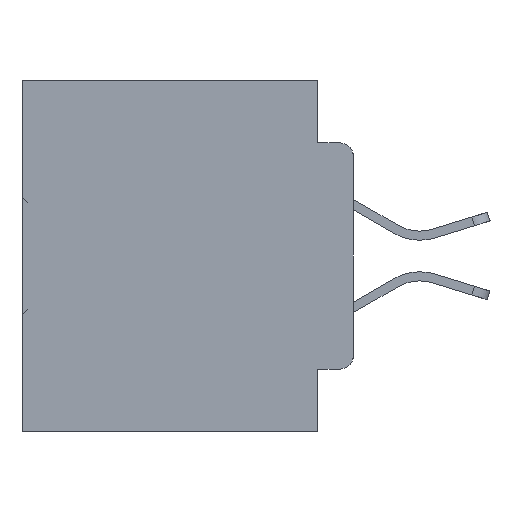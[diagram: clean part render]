
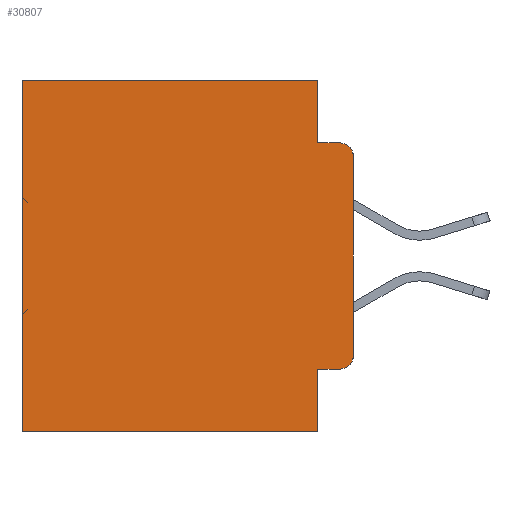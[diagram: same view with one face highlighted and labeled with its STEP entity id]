
A CAD part, left-side view. The second image highlights one B-rep face of the part: STEP entity #30807.
In plain terms, the highlighted planar face has unit normal (-1, 0, 0).
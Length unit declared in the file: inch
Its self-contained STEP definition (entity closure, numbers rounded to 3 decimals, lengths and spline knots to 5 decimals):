
#446 = CARTESIAN_POINT ( 'NONE',  ( 0.298, 0.051, -0.4115 ) ) ;
#1013 = VERTEX_POINT ( 'NONE', #8105 ) ;
#1316 = DIRECTION ( 'NONE',  ( 1., 0., 0. ) ) ;
#1449 = VECTOR ( 'NONE', #35092, 39.37008 ) ;
#1541 = EDGE_CURVE ( 'NONE', #20208, #4711, #32764, .T. ) ;
#1585 = VERTEX_POINT ( 'NONE', #5259 ) ;
#3361 = ORIENTED_EDGE ( 'NONE', *, *, #20859, .T. ) ;
#3576 = VECTOR ( 'NONE', #9005, 39.37008 ) ;
#4711 = VERTEX_POINT ( 'NONE', #33157 ) ;
#5133 = DIRECTION ( 'NONE',  ( 0., 1., 0. ) ) ;
#5152 = AXIS2_PLACEMENT_3D ( 'NONE', #24605, #1316, #24485 ) ;
#5259 = CARTESIAN_POINT ( 'NONE',  ( 0.298, 0.473, -0.5 ) ) ;
#5609 = VERTEX_POINT ( 'NONE', #18625 ) ;
#5916 = VECTOR ( 'NONE', #22371, 39.37008 ) ;
#7751 = LINE ( 'NONE', #8221, #5916 ) ;
#8022 = LINE ( 'NONE', #22755, #19784 ) ;
#8098 = EDGE_LOOP ( 'NONE', ( #30138, #3361, #35336, #16596, #19756, #23698, #16095, #12372, #8615, #29081 ) ) ;
#8105 = CARTESIAN_POINT ( 'NONE',  ( 0.298, 0., -0.3915 ) ) ;
#8221 = CARTESIAN_POINT ( 'NONE',  ( 0.298, 0.051, 0. ) ) ;
#8615 = ORIENTED_EDGE ( 'NONE', *, *, #26457, .T. ) ;
#9005 = DIRECTION ( 'NONE',  ( 0., 1., 0. ) ) ;
#9333 = DIRECTION ( 'NONE',  ( 0., -1., 0. ) ) ;
#9660 = LINE ( 'NONE', #446, #31742 ) ;
#10232 = EDGE_CURVE ( 'NONE', #5609, #1013, #26133, .T. ) ;
#11581 = EDGE_CURVE ( 'NONE', #22192, #26624, #8022, .T. ) ;
#12372 = ORIENTED_EDGE ( 'NONE', *, *, #14335, .F. ) ;
#12970 = DIRECTION ( 'NONE',  ( 0., 0., -1. ) ) ;
#13255 = DIRECTION ( 'NONE',  ( -1., 0., 0. ) ) ;
#13419 = VECTOR ( 'NONE', #12970, 39.37008 ) ;
#13526 = EDGE_CURVE ( 'NONE', #4711, #1585, #34059, .T. ) ;
#14335 = EDGE_CURVE ( 'NONE', #31553, #18210, #26596, .T. ) ;
#16095 = ORIENTED_EDGE ( 'NONE', *, *, #31212, .F. ) ;
#16596 = ORIENTED_EDGE ( 'NONE', *, *, #30222, .F. ) ;
#18210 = VERTEX_POINT ( 'NONE', #31781 ) ;
#18625 = CARTESIAN_POINT ( 'NONE',  ( 0.298, 0., -0.1085 ) ) ;
#19756 = ORIENTED_EDGE ( 'NONE', *, *, #1541, .T. ) ;
#19784 = VECTOR ( 'NONE', #31395, 39.37008 ) ;
#19881 = CARTESIAN_POINT ( 'NONE',  ( 0.298, 0.02, -0.3915 ) ) ;
#20208 = VERTEX_POINT ( 'NONE', #27887 ) ;
#20795 = CIRCLE ( 'NONE', #26571, 0.02 ) ;
#20859 = EDGE_CURVE ( 'NONE', #5609, #26624, #29845, .T. ) ;
#21051 = VERTEX_POINT ( 'NONE', #21909 ) ;
#21712 = PLANE ( 'NONE',  #5152 ) ;
#21909 = CARTESIAN_POINT ( 'NONE',  ( 0.298, 0.02, -0.4115 ) ) ;
#22051 = DIRECTION ( 'NONE',  ( 0., 0., -1. ) ) ;
#22192 = VERTEX_POINT ( 'NONE', #31010 ) ;
#22371 = DIRECTION ( 'NONE',  ( 0., 0., -1. ) ) ;
#22755 = CARTESIAN_POINT ( 'NONE',  ( 0.298, 0.051, -0.0885 ) ) ;
#23145 = DIRECTION ( 'NONE',  ( 0., 0., -1. ) ) ;
#23698 = ORIENTED_EDGE ( 'NONE', *, *, #13526, .T. ) ;
#24485 = DIRECTION ( 'NONE',  ( 0., 0., -1. ) ) ;
#24605 = CARTESIAN_POINT ( 'NONE',  ( 0.298, 0., 0. ) ) ;
#26133 = LINE ( 'NONE', #32671, #33326 ) ;
#26157 = AXIS2_PLACEMENT_3D ( 'NONE', #30437, #13255, #22051 ) ;
#26457 = EDGE_CURVE ( 'NONE', #31553, #21051, #9660, .T. ) ;
#26479 = VECTOR ( 'NONE', #5133, 39.37008 ) ;
#26571 = AXIS2_PLACEMENT_3D ( 'NONE', #19881, #31655, #23145 ) ;
#26596 = LINE ( 'NONE', #29352, #1449 ) ;
#26624 = VERTEX_POINT ( 'NONE', #32759 ) ;
#27887 = CARTESIAN_POINT ( 'NONE',  ( 0.298, 0.051, 0. ) ) ;
#28187 = CARTESIAN_POINT ( 'NONE',  ( 0.298, 0., 0. ) ) ;
#29081 = ORIENTED_EDGE ( 'NONE', *, *, #29639, .T. ) ;
#29287 = FACE_OUTER_BOUND ( 'NONE', #8098, .T. ) ;
#29352 = CARTESIAN_POINT ( 'NONE',  ( 0.298, 0.051, 0. ) ) ;
#29639 = EDGE_CURVE ( 'NONE', #21051, #1013, #20795, .T. ) ;
#29845 = CIRCLE ( 'NONE', #26157, 0.02 ) ;
#30138 = ORIENTED_EDGE ( 'NONE', *, *, #10232, .F. ) ;
#30171 = LINE ( 'NONE', #34557, #3576 ) ;
#30222 = EDGE_CURVE ( 'NONE', #20208, #22192, #7751, .T. ) ;
#30437 = CARTESIAN_POINT ( 'NONE',  ( 0.298, 0.02, -0.1085 ) ) ;
#30807 = ADVANCED_FACE ( 'NONE', ( #29287 ), #21712, .F. ) ;
#31010 = CARTESIAN_POINT ( 'NONE',  ( 0.298, 0.051, -0.0885 ) ) ;
#31212 = EDGE_CURVE ( 'NONE', #18210, #1585, #30171, .T. ) ;
#31395 = DIRECTION ( 'NONE',  ( 0., -1., 0. ) ) ;
#31553 = VERTEX_POINT ( 'NONE', #33933 ) ;
#31655 = DIRECTION ( 'NONE',  ( -1., 0., 0. ) ) ;
#31742 = VECTOR ( 'NONE', #9333, 39.37008 ) ;
#31781 = CARTESIAN_POINT ( 'NONE',  ( 0.298, 0.051, -0.5 ) ) ;
#32671 = CARTESIAN_POINT ( 'NONE',  ( 0.298, 0., 0. ) ) ;
#32759 = CARTESIAN_POINT ( 'NONE',  ( 0.298, 0.02, -0.0885 ) ) ;
#32764 = LINE ( 'NONE', #28187, #26479 ) ;
#33157 = CARTESIAN_POINT ( 'NONE',  ( 0.298, 0.473, 0. ) ) ;
#33326 = VECTOR ( 'NONE', #35419, 39.37008 ) ;
#33933 = CARTESIAN_POINT ( 'NONE',  ( 0.298, 0.051, -0.4115 ) ) ;
#34059 = LINE ( 'NONE', #35664, #13419 ) ;
#34557 = CARTESIAN_POINT ( 'NONE',  ( 0.298, 0., -0.5 ) ) ;
#35092 = DIRECTION ( 'NONE',  ( 0., 0., -1. ) ) ;
#35336 = ORIENTED_EDGE ( 'NONE', *, *, #11581, .F. ) ;
#35419 = DIRECTION ( 'NONE',  ( 0., 0., -1. ) ) ;
#35664 = CARTESIAN_POINT ( 'NONE',  ( 0.298, 0.473, 0. ) ) ;
